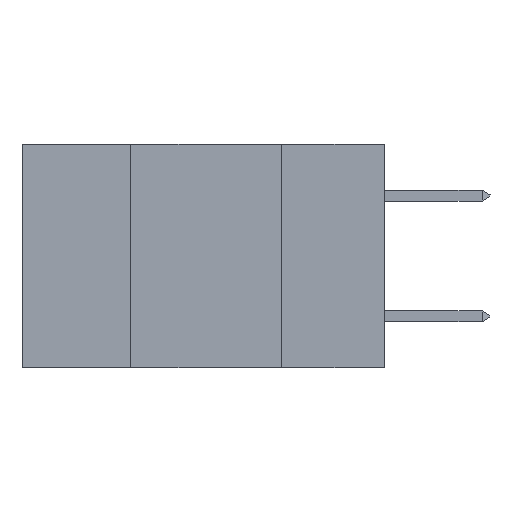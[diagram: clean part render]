
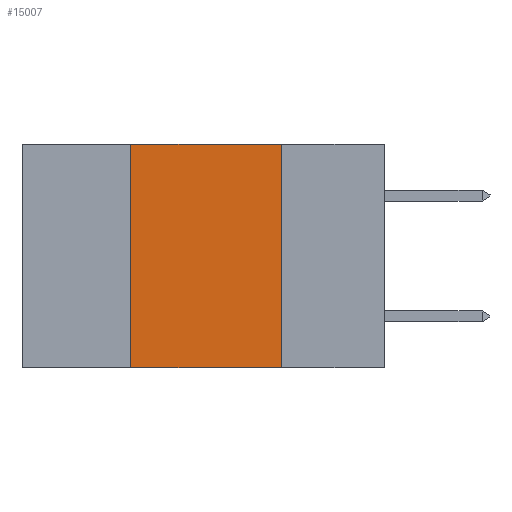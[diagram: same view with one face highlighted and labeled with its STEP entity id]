
A CAD part, left-side view. The second image highlights one B-rep face of the part: STEP entity #15007.
In plain terms, the highlighted planar face has unit normal (-1, 0, 0).
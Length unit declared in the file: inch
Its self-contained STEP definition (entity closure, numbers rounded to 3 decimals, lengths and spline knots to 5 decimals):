
#614 = VERTEX_POINT ( 'NONE', #8611 ) ;
#973 = CARTESIAN_POINT ( 'NONE',  ( 0., 0.42, -0.37 ) ) ;
#978 = VERTEX_POINT ( 'NONE', #25608 ) ;
#2062 = LINE ( 'NONE', #12645, #32385 ) ;
#2423 = ORIENTED_EDGE ( 'NONE', *, *, #7778, .T. ) ;
#2973 = CARTESIAN_POINT ( 'NONE',  ( 0., 0.17, -0.37 ) ) ;
#3044 = VERTEX_POINT ( 'NONE', #2973 ) ;
#3462 = DIRECTION ( 'NONE',  ( 0., 0., -1. ) ) ;
#4946 = ORIENTED_EDGE ( 'NONE', *, *, #33117, .F. ) ;
#6100 = VECTOR ( 'NONE', #27308, 39.37008 ) ;
#6467 = CARTESIAN_POINT ( 'NONE',  ( 0., 0.17, 0. ) ) ;
#7778 = EDGE_CURVE ( 'NONE', #7845, #3044, #15464, .T. ) ;
#7845 = VERTEX_POINT ( 'NONE', #973 ) ;
#8611 = CARTESIAN_POINT ( 'NONE',  ( 0., 0.42, 0. ) ) ;
#9297 = FACE_OUTER_BOUND ( 'NONE', #9406, .T. ) ;
#9406 = EDGE_LOOP ( 'NONE', ( #31480, #4946, #11817, #2423 ) ) ;
#11132 = CARTESIAN_POINT ( 'NONE',  ( 0., 0.42, 0. ) ) ;
#11817 = ORIENTED_EDGE ( 'NONE', *, *, #12240, .F. ) ;
#12240 = EDGE_CURVE ( 'NONE', #7845, #614, #15627, .T. ) ;
#12645 = CARTESIAN_POINT ( 'NONE',  ( 0., 0.6, 0. ) ) ;
#13981 = CARTESIAN_POINT ( 'NONE',  ( 0., 0.6, -0.37 ) ) ;
#15007 = ADVANCED_FACE ( 'NONE', ( #9297 ), #19146, .F. ) ;
#15464 = LINE ( 'NONE', #13981, #6100 ) ;
#15627 = LINE ( 'NONE', #11132, #25141 ) ;
#19146 = PLANE ( 'NONE',  #29391 ) ;
#21678 = DIRECTION ( 'NONE',  ( 1., 0., 0. ) ) ;
#22936 = EDGE_CURVE ( 'NONE', #978, #3044, #30706, .T. ) ;
#25141 = VECTOR ( 'NONE', #27665, 39.37008 ) ;
#25608 = CARTESIAN_POINT ( 'NONE',  ( 0., 0.17, 0. ) ) ;
#26642 = VECTOR ( 'NONE', #29817, 39.37008 ) ;
#27308 = DIRECTION ( 'NONE',  ( 0., -1., 0. ) ) ;
#27665 = DIRECTION ( 'NONE',  ( 0., 0., 1. ) ) ;
#29391 = AXIS2_PLACEMENT_3D ( 'NONE', #32281, #21678, #3462 ) ;
#29817 = DIRECTION ( 'NONE',  ( 0., 0., -1. ) ) ;
#30706 = LINE ( 'NONE', #6467, #26642 ) ;
#31077 = DIRECTION ( 'NONE',  ( 0., -1., 0. ) ) ;
#31480 = ORIENTED_EDGE ( 'NONE', *, *, #22936, .F. ) ;
#32281 = CARTESIAN_POINT ( 'NONE',  ( 0., 0.6, 0. ) ) ;
#32385 = VECTOR ( 'NONE', #31077, 39.37008 ) ;
#33117 = EDGE_CURVE ( 'NONE', #614, #978, #2062, .T. ) ;
